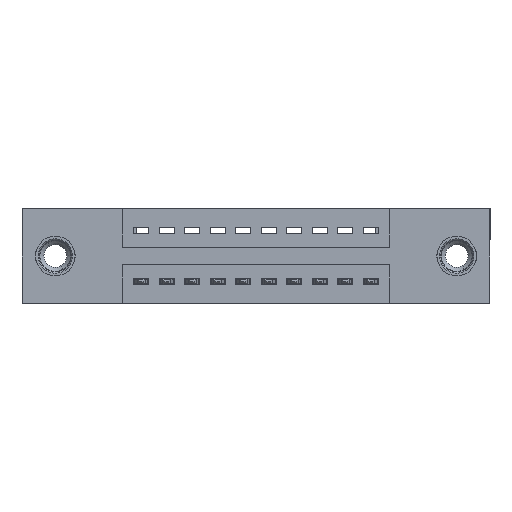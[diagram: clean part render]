
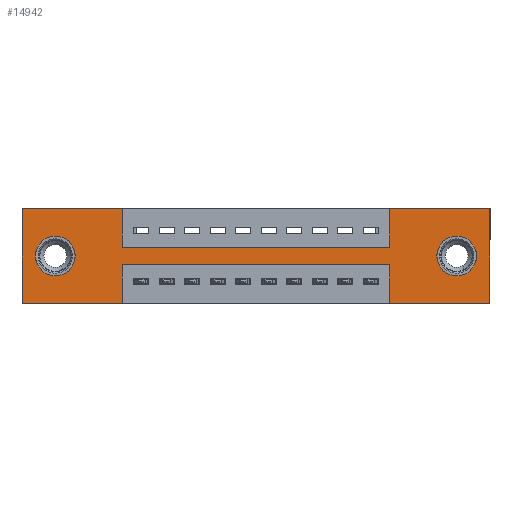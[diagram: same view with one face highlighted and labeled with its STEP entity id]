
A CAD part, front view. The second image highlights one B-rep face of the part: STEP entity #14942.
In plain terms, the highlighted planar face has unit normal (0, -1, 0).
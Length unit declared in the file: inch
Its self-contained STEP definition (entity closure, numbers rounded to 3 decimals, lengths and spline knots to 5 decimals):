
#25 = VERTEX_POINT ( 'NONE', #548 ) ;
#29 = DIRECTION ( 'NONE',  ( 0., 0., 1. ) ) ;
#154 = CARTESIAN_POINT ( 'NONE',  ( 1.835, 0., 0. ) ) ;
#191 = EDGE_CURVE ( 'NONE', #13447, #7070, #2512, .T. ) ;
#297 = DIRECTION ( 'NONE',  ( 0., 0., -1. ) ) ;
#317 = ORIENTED_EDGE ( 'NONE', *, *, #3313, .F. ) ;
#338 = DIRECTION ( 'NONE',  ( 0., 0., 1. ) ) ;
#548 = CARTESIAN_POINT ( 'NONE',  ( 1.4425, 0., -0.22 ) ) ;
#549 = LINE ( 'NONE', #5732, #4961 ) ;
#618 = FACE_BOUND ( 'NONE', #3620, .T. ) ;
#827 = CARTESIAN_POINT ( 'NONE',  ( 1.705, 0., -0.185 ) ) ;
#891 = CARTESIAN_POINT ( 'NONE',  ( 0., 0., 0. ) ) ;
#1344 = ORIENTED_EDGE ( 'NONE', *, *, #2039, .F. ) ;
#1615 = ORIENTED_EDGE ( 'NONE', *, *, #2711, .F. ) ;
#1737 = ORIENTED_EDGE ( 'NONE', *, *, #3564, .F. ) ;
#1809 = CARTESIAN_POINT ( 'NONE',  ( 0.13, 0., -0.263 ) ) ;
#1874 = LINE ( 'NONE', #891, #12727 ) ;
#1974 = DIRECTION ( 'NONE',  ( -1., 0., 0. ) ) ;
#1995 = VERTEX_POINT ( 'NONE', #16635 ) ;
#2018 = CARTESIAN_POINT ( 'NONE',  ( 1.705, 0., -0.107 ) ) ;
#2039 = EDGE_CURVE ( 'NONE', #11389, #7398, #14764, .T. ) ;
#2512 = CIRCLE ( 'NONE', #15564, 0.078 ) ;
#2581 = DIRECTION ( 'NONE',  ( 0., -1., 0. ) ) ;
#2639 = FACE_OUTER_BOUND ( 'NONE', #2885, .T. ) ;
#2711 = EDGE_CURVE ( 'NONE', #2800, #11389, #14540, .T. ) ;
#2761 = CARTESIAN_POINT ( 'NONE',  ( 0., 0., 0. ) ) ;
#2800 = VERTEX_POINT ( 'NONE', #15237 ) ;
#2885 = EDGE_LOOP ( 'NONE', ( #14978, #16600, #14445, #14779, #1344, #1615, #13123, #1737, #317, #16713, #10691, #6915 ) ) ;
#3017 = VERTEX_POINT ( 'NONE', #8641 ) ;
#3035 = EDGE_CURVE ( 'NONE', #7398, #3017, #9312, .T. ) ;
#3248 = VECTOR ( 'NONE', #15252, 39.37008 ) ;
#3313 = EDGE_CURVE ( 'NONE', #5655, #8129, #10903, .T. ) ;
#3447 = CIRCLE ( 'NONE', #10226, 0.078 ) ;
#3564 = EDGE_CURVE ( 'NONE', #8129, #11198, #7108, .T. ) ;
#3620 = EDGE_LOOP ( 'NONE', ( #16615, #7744 ) ) ;
#3638 = DIRECTION ( 'NONE',  ( 1., 0., 0. ) ) ;
#3835 = CARTESIAN_POINT ( 'NONE',  ( 1.835, 0., -0.37 ) ) ;
#4238 = ORIENTED_EDGE ( 'NONE', *, *, #14822, .T. ) ;
#4264 = EDGE_CURVE ( 'NONE', #3017, #25, #14696, .T. ) ;
#4406 = VECTOR ( 'NONE', #6491, 39.37008 ) ;
#4527 = EDGE_CURVE ( 'NONE', #25, #1995, #6220, .T. ) ;
#4620 = DIRECTION ( 'NONE',  ( 0., 1., 0. ) ) ;
#4718 = CARTESIAN_POINT ( 'NONE',  ( 1.4425, 0., -0.15 ) ) ;
#4797 = CARTESIAN_POINT ( 'NONE',  ( 0., 0., -0.37 ) ) ;
#4961 = VECTOR ( 'NONE', #14735, 39.37008 ) ;
#5036 = DIRECTION ( 'NONE',  ( 0., 1., 0. ) ) ;
#5313 = CARTESIAN_POINT ( 'NONE',  ( 0.13, 0., -0.107 ) ) ;
#5378 = AXIS2_PLACEMENT_3D ( 'NONE', #13542, #4620, #8453 ) ;
#5434 = EDGE_CURVE ( 'NONE', #12266, #14234, #10233, .T. ) ;
#5655 = VERTEX_POINT ( 'NONE', #5768 ) ;
#5732 = CARTESIAN_POINT ( 'NONE',  ( 0.3925, 0., -0.37 ) ) ;
#5768 = CARTESIAN_POINT ( 'NONE',  ( 0.3925, 0., 0. ) ) ;
#6074 = FACE_BOUND ( 'NONE', #13461, .T. ) ;
#6220 = LINE ( 'NONE', #9730, #14874 ) ;
#6264 = CARTESIAN_POINT ( 'NONE',  ( 0., 0., 0. ) ) ;
#6270 = CIRCLE ( 'NONE', #5378, 0.078 ) ;
#6472 = LINE ( 'NONE', #6960, #11291 ) ;
#6491 = DIRECTION ( 'NONE',  ( 0., 0., 1. ) ) ;
#6555 = CARTESIAN_POINT ( 'NONE',  ( 0.13, 0., -0.185 ) ) ;
#6610 = DIRECTION ( 'NONE',  ( 0., 0., -1. ) ) ;
#6692 = CARTESIAN_POINT ( 'NONE',  ( 0.3925, 0., -0.37 ) ) ;
#6795 = VERTEX_POINT ( 'NONE', #5313 ) ;
#6915 = ORIENTED_EDGE ( 'NONE', *, *, #15136, .F. ) ;
#6960 = CARTESIAN_POINT ( 'NONE',  ( 0., 0., -0.37 ) ) ;
#7012 = AXIS2_PLACEMENT_3D ( 'NONE', #16714, #2581, #297 ) ;
#7070 = VERTEX_POINT ( 'NONE', #16362 ) ;
#7108 = LINE ( 'NONE', #14836, #13300 ) ;
#7145 = DIRECTION ( 'NONE',  ( 0., 0., -1. ) ) ;
#7398 = VERTEX_POINT ( 'NONE', #3835 ) ;
#7444 = DIRECTION ( 'NONE',  ( 0., 0., -1. ) ) ;
#7654 = DIRECTION ( 'NONE',  ( 0., 0., 1. ) ) ;
#7744 = ORIENTED_EDGE ( 'NONE', *, *, #14816, .T. ) ;
#8129 = VERTEX_POINT ( 'NONE', #9679 ) ;
#8224 = EDGE_CURVE ( 'NONE', #1995, #8809, #549, .T. ) ;
#8427 = VERTEX_POINT ( 'NONE', #1809 ) ;
#8453 = DIRECTION ( 'NONE',  ( 0., 0., 1. ) ) ;
#8641 = CARTESIAN_POINT ( 'NONE',  ( 1.4425, 0., -0.37 ) ) ;
#8645 = EDGE_CURVE ( 'NONE', #11198, #2800, #16078, .T. ) ;
#8809 = VERTEX_POINT ( 'NONE', #6692 ) ;
#8901 = DIRECTION ( 'NONE',  ( -1., 0., 0. ) ) ;
#9312 = LINE ( 'NONE', #4797, #14727 ) ;
#9679 = CARTESIAN_POINT ( 'NONE',  ( 0.3925, 0., -0.15 ) ) ;
#9730 = CARTESIAN_POINT ( 'NONE',  ( 0.3925, 0., -0.22 ) ) ;
#9866 = VECTOR ( 'NONE', #338, 39.37008 ) ;
#9913 = CARTESIAN_POINT ( 'NONE',  ( 0.3925, 0., 0. ) ) ;
#10087 = ORIENTED_EDGE ( 'NONE', *, *, #12057, .T. ) ;
#10226 = AXIS2_PLACEMENT_3D ( 'NONE', #14290, #12918, #6610 ) ;
#10233 = LINE ( 'NONE', #2761, #12420 ) ;
#10691 = ORIENTED_EDGE ( 'NONE', *, *, #5434, .F. ) ;
#10699 = CARTESIAN_POINT ( 'NONE',  ( 1.835, 0., 0. ) ) ;
#10903 = LINE ( 'NONE', #9913, #14521 ) ;
#11020 = DIRECTION ( 'NONE',  ( 1., 0., 0. ) ) ;
#11057 = EDGE_CURVE ( 'NONE', #14234, #5655, #1874, .T. ) ;
#11142 = DIRECTION ( 'NONE',  ( 0., 1., 0. ) ) ;
#11198 = VERTEX_POINT ( 'NONE', #4718 ) ;
#11291 = VECTOR ( 'NONE', #12093, 39.37008 ) ;
#11389 = VERTEX_POINT ( 'NONE', #10699 ) ;
#11657 = CARTESIAN_POINT ( 'NONE',  ( 1.4425, 0., -0.37 ) ) ;
#11709 = CIRCLE ( 'NONE', #14723, 0.078 ) ;
#12057 = EDGE_CURVE ( 'NONE', #6795, #8427, #6270, .T. ) ;
#12093 = DIRECTION ( 'NONE',  ( -1., 0., 0. ) ) ;
#12266 = VERTEX_POINT ( 'NONE', #15474 ) ;
#12420 = VECTOR ( 'NONE', #29, 39.37008 ) ;
#12727 = VECTOR ( 'NONE', #3638, 39.37008 ) ;
#12918 = DIRECTION ( 'NONE',  ( 0., 1., 0. ) ) ;
#12976 = PLANE ( 'NONE',  #7012 ) ;
#13073 = DIRECTION ( 'NONE',  ( 0., 0., -1. ) ) ;
#13117 = CARTESIAN_POINT ( 'NONE',  ( 0., 0., 0. ) ) ;
#13123 = ORIENTED_EDGE ( 'NONE', *, *, #8645, .F. ) ;
#13198 = CARTESIAN_POINT ( 'NONE',  ( 1.4425, 0., 0. ) ) ;
#13300 = VECTOR ( 'NONE', #11020, 39.37008 ) ;
#13447 = VERTEX_POINT ( 'NONE', #2018 ) ;
#13461 = EDGE_LOOP ( 'NONE', ( #10087, #4238 ) ) ;
#13542 = CARTESIAN_POINT ( 'NONE',  ( 0.13, 0., -0.185 ) ) ;
#14234 = VERTEX_POINT ( 'NONE', #13117 ) ;
#14290 = CARTESIAN_POINT ( 'NONE',  ( 1.705, 0., -0.185 ) ) ;
#14445 = ORIENTED_EDGE ( 'NONE', *, *, #4264, .F. ) ;
#14521 = VECTOR ( 'NONE', #7444, 39.37008 ) ;
#14540 = LINE ( 'NONE', #6264, #3248 ) ;
#14696 = LINE ( 'NONE', #11657, #4406 ) ;
#14723 = AXIS2_PLACEMENT_3D ( 'NONE', #6555, #5036, #7654 ) ;
#14727 = VECTOR ( 'NONE', #8901, 39.37008 ) ;
#14735 = DIRECTION ( 'NONE',  ( 0., 0., -1. ) ) ;
#14764 = LINE ( 'NONE', #154, #15545 ) ;
#14779 = ORIENTED_EDGE ( 'NONE', *, *, #3035, .F. ) ;
#14816 = EDGE_CURVE ( 'NONE', #7070, #13447, #3447, .T. ) ;
#14822 = EDGE_CURVE ( 'NONE', #8427, #6795, #11709, .T. ) ;
#14836 = CARTESIAN_POINT ( 'NONE',  ( 0.3925, 0., -0.15 ) ) ;
#14874 = VECTOR ( 'NONE', #1974, 39.37008 ) ;
#14942 = ADVANCED_FACE ( 'NONE', ( #618, #6074, #2639 ), #12976, .T. ) ;
#14978 = ORIENTED_EDGE ( 'NONE', *, *, #8224, .F. ) ;
#15136 = EDGE_CURVE ( 'NONE', #8809, #12266, #6472, .T. ) ;
#15237 = CARTESIAN_POINT ( 'NONE',  ( 1.4425, 0., 0. ) ) ;
#15252 = DIRECTION ( 'NONE',  ( 1., 0., 0. ) ) ;
#15474 = CARTESIAN_POINT ( 'NONE',  ( 0., 0., -0.37 ) ) ;
#15545 = VECTOR ( 'NONE', #13073, 39.37008 ) ;
#15564 = AXIS2_PLACEMENT_3D ( 'NONE', #827, #11142, #7145 ) ;
#16078 = LINE ( 'NONE', #13198, #9866 ) ;
#16362 = CARTESIAN_POINT ( 'NONE',  ( 1.705, 0., -0.263 ) ) ;
#16600 = ORIENTED_EDGE ( 'NONE', *, *, #4527, .F. ) ;
#16615 = ORIENTED_EDGE ( 'NONE', *, *, #191, .T. ) ;
#16635 = CARTESIAN_POINT ( 'NONE',  ( 0.3925, 0., -0.22 ) ) ;
#16713 = ORIENTED_EDGE ( 'NONE', *, *, #11057, .F. ) ;
#16714 = CARTESIAN_POINT ( 'NONE',  ( 0., 0., -0.37 ) ) ;
